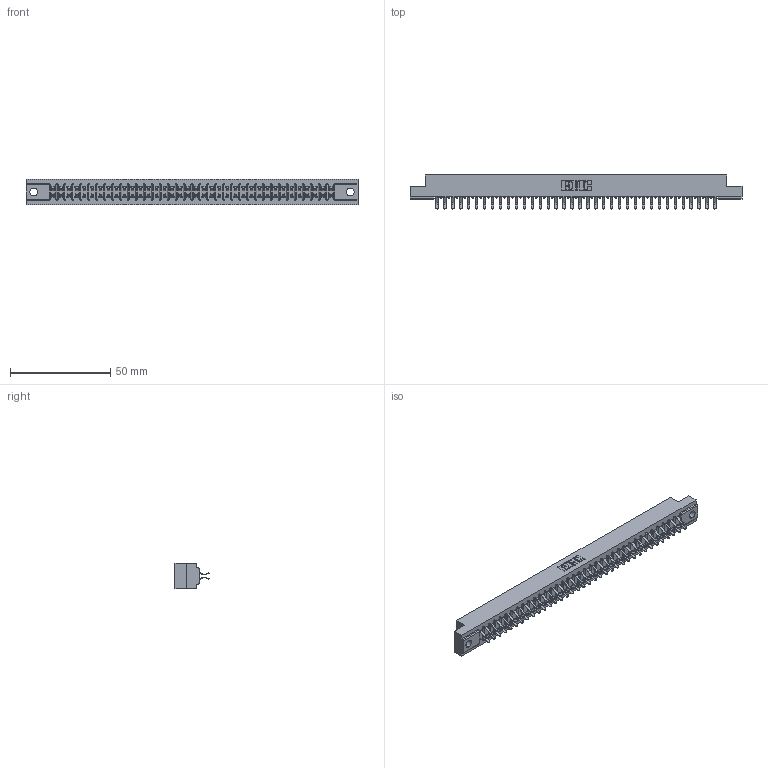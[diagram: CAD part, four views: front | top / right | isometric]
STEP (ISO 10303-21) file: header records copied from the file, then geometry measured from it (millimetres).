
FILE_DESCRIPTION (( 'STEP AP203' ), '1' );
FILE_NAME ('357-072-556-202.STEP', '2019-09-19T11:39:20', ( '' ), ( '' ), 'SwSTEP 2.0', 'SolidWorks 2016', '' );
FILE_SCHEMA (( 'CONFIG_CONTROL_DESIGN' ));
Length unit declared in the file: inch
Products named in the file (3): 307-290-001_556; 307 Part_.128 Dia Mounting Holes; 357-072-556-202
Assembly tree (73 placements, depth 2):
  357-072-556-202
    307 Part_.128 Dia Mounting Holes
    307-290-001_556  x72
Bounding box: 165.66 x 16.97 x 12.7 mm (x, y, z)
Volume: 17472.4 mm3; surface area: 20869.4 mm2
Topology: 73 solids, 73 shells, 3755 faces, 10547 edges, 6834 vertices
Faces by surface type: plane 2446, cylinder 1235, sphere 74
Entity records: 32860 total; most frequent: CARTESIAN_POINT 5376, ORIENTED_EDGE 5326, DIRECTION 5269, EDGE_CURVE 2663, LINE 2039, VECTOR 2039, VERTEX_POINT 1722, AXIS2_PLACEMENT_3D 1615
